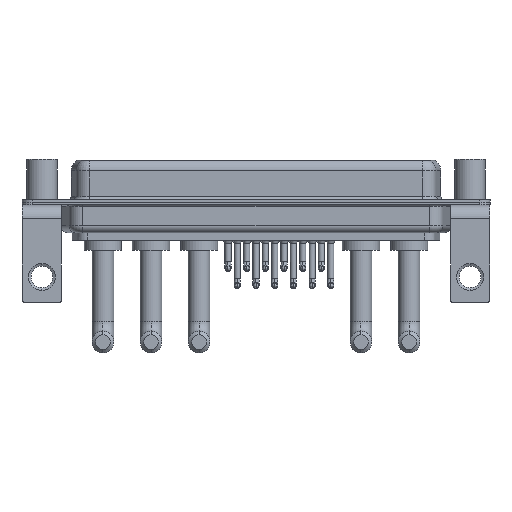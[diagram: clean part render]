
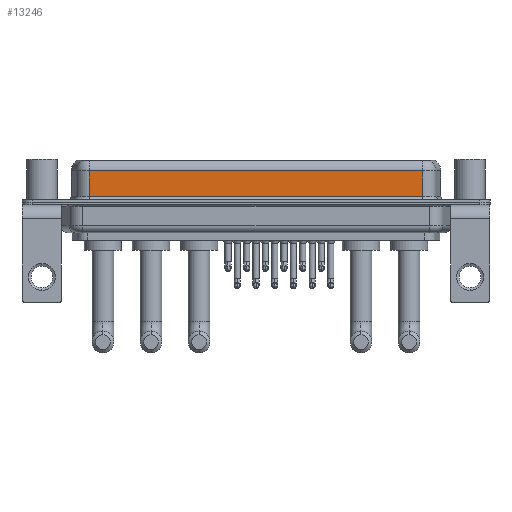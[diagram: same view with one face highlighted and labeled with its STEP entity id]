
A CAD part, front view. The second image highlights one B-rep face of the part: STEP entity #13246.
In plain terms, the highlighted planar face has unit normal (0, -1, 0).
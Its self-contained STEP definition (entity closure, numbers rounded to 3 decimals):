
#12 = LINE ( 'NONE', #21161, #8350 ) ;
#201 = EDGE_CURVE ( 'NONE', #22085, #16115, #12, .T. ) ;
#1352 = DIRECTION ( 'NONE',  ( 0., 0., -1. ) ) ;
#1381 = AXIS2_PLACEMENT_3D ( 'NONE', #20199, #18471, #7779 ) ;
#1532 = VECTOR ( 'NONE', #9116, 1000. ) ;
#2041 = CARTESIAN_POINT ( 'NONE',  ( 56.462, -3.95, 4.65 ) ) ;
#2303 = VECTOR ( 'NONE', #15961, 1000. ) ;
#2600 = FACE_OUTER_BOUND ( 'NONE', #13751, .T. ) ;
#2676 = ORIENTED_EDGE ( 'NONE', *, *, #17904, .F. ) ;
#2785 = ORIENTED_EDGE ( 'NONE', *, *, #7666, .T. ) ;
#2972 = ORIENTED_EDGE ( 'NONE', *, *, #5955, .T. ) ;
#3091 = LINE ( 'NONE', #10099, #17481 ) ;
#4086 = PLANE ( 'NONE',  #1381 ) ;
#4909 = CARTESIAN_POINT ( 'NONE',  ( 7.038, -3.95, 0.9 ) ) ;
#5955 = EDGE_CURVE ( 'NONE', #21771, #19151, #15900, .T. ) ;
#7666 = EDGE_CURVE ( 'NONE', #19151, #22085, #12064, .T. ) ;
#7779 = DIRECTION ( 'NONE',  ( 0., 0., 1. ) ) ;
#8350 = VECTOR ( 'NONE', #17716, 1000. ) ;
#9116 = DIRECTION ( 'NONE',  ( -1., 0., 0. ) ) ;
#9785 = CARTESIAN_POINT ( 'NONE',  ( 7.038, -3.95, 4.65 ) ) ;
#10099 = CARTESIAN_POINT ( 'NONE',  ( 56.462, -3.95, 6.4 ) ) ;
#10827 = CARTESIAN_POINT ( 'NONE',  ( 56.462, -3.95, 4.65 ) ) ;
#12064 = LINE ( 'NONE', #19085, #2303 ) ;
#13246 = ADVANCED_FACE ( 'NONE', ( #2600 ), #4086, .F. ) ;
#13751 = EDGE_LOOP ( 'NONE', ( #2676, #2972, #2785, #22443 ) ) ;
#15900 = LINE ( 'NONE', #10827, #1532 ) ;
#15961 = DIRECTION ( 'NONE',  ( 0., 0., -1. ) ) ;
#16115 = VERTEX_POINT ( 'NONE', #18050 ) ;
#17481 = VECTOR ( 'NONE', #1352, 1000. ) ;
#17716 = DIRECTION ( 'NONE',  ( 1., 0., 0. ) ) ;
#17904 = EDGE_CURVE ( 'NONE', #21771, #16115, #3091, .T. ) ;
#18050 = CARTESIAN_POINT ( 'NONE',  ( 56.462, -3.95, 0.9 ) ) ;
#18471 = DIRECTION ( 'NONE',  ( 0., 1., 0. ) ) ;
#19085 = CARTESIAN_POINT ( 'NONE',  ( 7.038, -3.95, 6.4 ) ) ;
#19151 = VERTEX_POINT ( 'NONE', #9785 ) ;
#20199 = CARTESIAN_POINT ( 'NONE',  ( 56.462, -3.95, 6.4 ) ) ;
#21161 = CARTESIAN_POINT ( 'NONE',  ( 56.462, -3.95, 0.9 ) ) ;
#21771 = VERTEX_POINT ( 'NONE', #2041 ) ;
#22085 = VERTEX_POINT ( 'NONE', #4909 ) ;
#22443 = ORIENTED_EDGE ( 'NONE', *, *, #201, .T. ) ;
